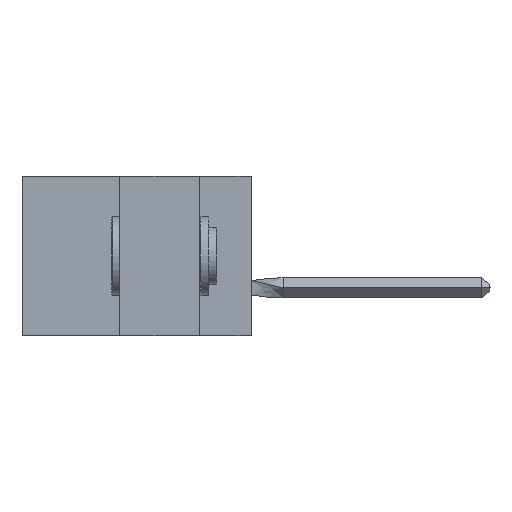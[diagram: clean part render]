
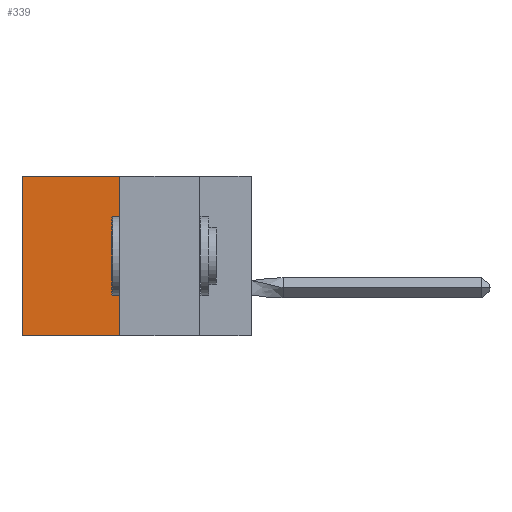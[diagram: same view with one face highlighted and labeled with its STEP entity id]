
A CAD part, left-side view. The second image highlights one B-rep face of the part: STEP entity #339.
In plain terms, the highlighted planar face has unit normal (-1, 0, 0).
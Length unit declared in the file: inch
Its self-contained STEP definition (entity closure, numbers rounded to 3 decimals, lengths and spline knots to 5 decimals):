
#339 = ADVANCED_FACE ( 'NONE', ( #14991 ), #17336, .F. ) ;
#501 = EDGE_CURVE ( 'NONE', #9002, #5125, #18912, .T. ) ;
#603 = CARTESIAN_POINT ( 'NONE',  ( 0.305, 0.413, 0. ) ) ;
#929 = DIRECTION ( 'NONE',  ( 0., 1., 0. ) ) ;
#1624 = DIRECTION ( 'NONE',  ( 0., 0., -1. ) ) ;
#2764 = EDGE_CURVE ( 'NONE', #19565, #9002, #17391, .T. ) ;
#2846 = CARTESIAN_POINT ( 'NONE',  ( 0.305, 0.72, 0. ) ) ;
#4255 = ORIENTED_EDGE ( 'NONE', *, *, #501, .T. ) ;
#4313 = LINE ( 'NONE', #8908, #9344 ) ;
#5125 = VERTEX_POINT ( 'NONE', #5252 ) ;
#5252 = CARTESIAN_POINT ( 'NONE',  ( 0.305, 0.72, -0.5 ) ) ;
#5654 = VERTEX_POINT ( 'NONE', #15788 ) ;
#6681 = CARTESIAN_POINT ( 'NONE',  ( 0.305, 0.413, -0.5 ) ) ;
#7235 = VECTOR ( 'NONE', #13166, 39.37008 ) ;
#7554 = CARTESIAN_POINT ( 'NONE',  ( 0.305, 0.413, 0. ) ) ;
#8405 = DIRECTION ( 'NONE',  ( 0., 0., -1. ) ) ;
#8908 = CARTESIAN_POINT ( 'NONE',  ( 0.305, 0.413, -0.5 ) ) ;
#9002 = VERTEX_POINT ( 'NONE', #2846 ) ;
#9344 = VECTOR ( 'NONE', #14294, 39.37008 ) ;
#9417 = ORIENTED_EDGE ( 'NONE', *, *, #21365, .F. ) ;
#9701 = EDGE_LOOP ( 'NONE', ( #4255, #21942, #9417, #11831 ) ) ;
#10551 = VECTOR ( 'NONE', #929, 39.37008 ) ;
#11831 = ORIENTED_EDGE ( 'NONE', *, *, #2764, .T. ) ;
#13100 = EDGE_CURVE ( 'NONE', #5654, #5125, #20711, .T. ) ;
#13166 = DIRECTION ( 'NONE',  ( 0., 1., 0. ) ) ;
#14108 = VECTOR ( 'NONE', #1624, 39.37008 ) ;
#14294 = DIRECTION ( 'NONE',  ( 0., 0., -1. ) ) ;
#14991 = FACE_OUTER_BOUND ( 'NONE', #9701, .T. ) ;
#15788 = CARTESIAN_POINT ( 'NONE',  ( 0.305, 0.413, -0.5 ) ) ;
#15981 = AXIS2_PLACEMENT_3D ( 'NONE', #6681, #22992, #8405 ) ;
#16294 = CARTESIAN_POINT ( 'NONE',  ( 0.305, 0.72, -0.5 ) ) ;
#17336 = PLANE ( 'NONE',  #15981 ) ;
#17391 = LINE ( 'NONE', #7554, #7235 ) ;
#18912 = LINE ( 'NONE', #16294, #14108 ) ;
#19065 = CARTESIAN_POINT ( 'NONE',  ( 0.305, 0.413, -0.5 ) ) ;
#19565 = VERTEX_POINT ( 'NONE', #603 ) ;
#20711 = LINE ( 'NONE', #19065, #10551 ) ;
#21365 = EDGE_CURVE ( 'NONE', #19565, #5654, #4313, .T. ) ;
#21942 = ORIENTED_EDGE ( 'NONE', *, *, #13100, .F. ) ;
#22992 = DIRECTION ( 'NONE',  ( 1., 0., 0. ) ) ;
